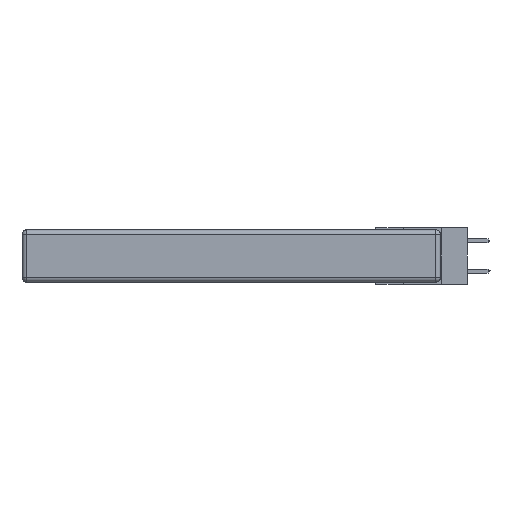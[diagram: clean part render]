
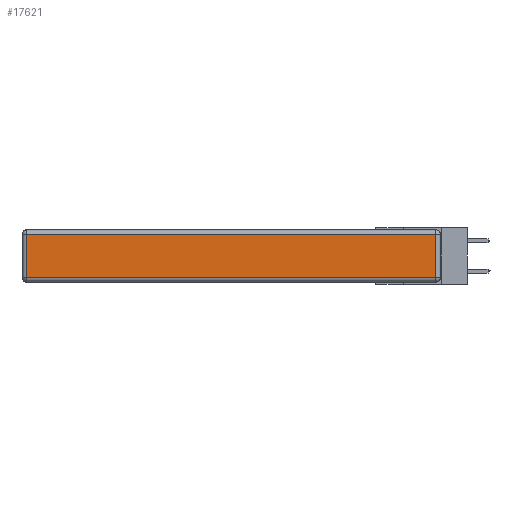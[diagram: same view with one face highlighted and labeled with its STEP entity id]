
A CAD part, left-side view. The second image highlights one B-rep face of the part: STEP entity #17621.
In plain terms, the highlighted planar face has unit normal (-1, 0, 0).
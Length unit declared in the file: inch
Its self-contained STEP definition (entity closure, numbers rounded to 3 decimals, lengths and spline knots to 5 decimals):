
#266 = DIRECTION ( 'NONE',  ( 0., 0., -1. ) ) ;
#439 = VECTOR ( 'NONE', #266, 39.37008 ) ;
#1260 = VERTEX_POINT ( 'NONE', #9912 ) ;
#2400 = EDGE_CURVE ( 'NONE', #16510, #3111, #18819, .T. ) ;
#2580 = EDGE_CURVE ( 'NONE', #1260, #16859, #7875, .T. ) ;
#3005 = CARTESIAN_POINT ( 'NONE',  ( 0., 0.03, -0.313 ) ) ;
#3111 = VERTEX_POINT ( 'NONE', #24826 ) ;
#4024 = CARTESIAN_POINT ( 'NONE',  ( 0., 2.72, -0.313 ) ) ;
#4674 = EDGE_LOOP ( 'NONE', ( #17686, #25148, #25658, #22364 ) ) ;
#7280 = CARTESIAN_POINT ( 'NONE',  ( 0., 0., -0.313 ) ) ;
#7875 = LINE ( 'NONE', #18034, #439 ) ;
#8492 = DIRECTION ( 'NONE',  ( -1., 0., 0. ) ) ;
#9380 = VECTOR ( 'NONE', #11870, 39.37008 ) ;
#9562 = CARTESIAN_POINT ( 'NONE',  ( 0., 0.03, -0.343 ) ) ;
#9912 = CARTESIAN_POINT ( 'NONE',  ( 0., 2.72, -0.03 ) ) ;
#10081 = EDGE_CURVE ( 'NONE', #3111, #1260, #16592, .T. ) ;
#10292 = VECTOR ( 'NONE', #23160, 39.37008 ) ;
#11714 = CARTESIAN_POINT ( 'NONE',  ( 0., 2.75, -0.03 ) ) ;
#11870 = DIRECTION ( 'NONE',  ( 0., 1., 0. ) ) ;
#12536 = DIRECTION ( 'NONE',  ( 0., 0., 1. ) ) ;
#13644 = AXIS2_PLACEMENT_3D ( 'NONE', #16783, #8492, #12536 ) ;
#14609 = PLANE ( 'NONE',  #13644 ) ;
#16311 = VECTOR ( 'NONE', #19597, 39.37008 ) ;
#16510 = VERTEX_POINT ( 'NONE', #3005 ) ;
#16592 = LINE ( 'NONE', #11714, #9380 ) ;
#16783 = CARTESIAN_POINT ( 'NONE',  ( 0., 0., -0.343 ) ) ;
#16859 = VERTEX_POINT ( 'NONE', #4024 ) ;
#17621 = ADVANCED_FACE ( 'NONE', ( #19361 ), #14609, .T. ) ;
#17686 = ORIENTED_EDGE ( 'NONE', *, *, #18251, .T. ) ;
#18034 = CARTESIAN_POINT ( 'NONE',  ( 0., 2.72, -0.343 ) ) ;
#18251 = EDGE_CURVE ( 'NONE', #16859, #16510, #21217, .T. ) ;
#18819 = LINE ( 'NONE', #9562, #16311 ) ;
#19361 = FACE_OUTER_BOUND ( 'NONE', #4674, .T. ) ;
#19597 = DIRECTION ( 'NONE',  ( 0., 0., 1. ) ) ;
#21217 = LINE ( 'NONE', #7280, #10292 ) ;
#22364 = ORIENTED_EDGE ( 'NONE', *, *, #2580, .T. ) ;
#23160 = DIRECTION ( 'NONE',  ( 0., -1., 0. ) ) ;
#24826 = CARTESIAN_POINT ( 'NONE',  ( 0., 0.03, -0.03 ) ) ;
#25148 = ORIENTED_EDGE ( 'NONE', *, *, #2400, .T. ) ;
#25658 = ORIENTED_EDGE ( 'NONE', *, *, #10081, .T. ) ;
